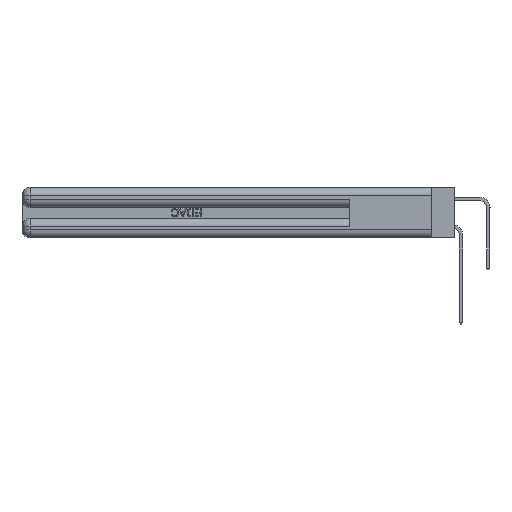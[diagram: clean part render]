
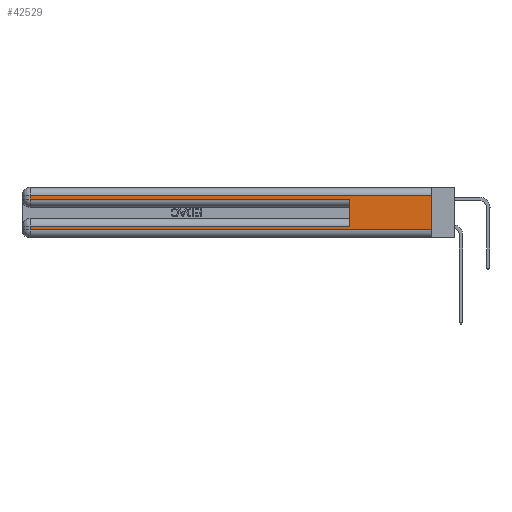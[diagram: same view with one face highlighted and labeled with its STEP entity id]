
A CAD part, left-side view. The second image highlights one B-rep face of the part: STEP entity #42529.
In plain terms, the highlighted planar face has unit normal (-1, 0, 0).
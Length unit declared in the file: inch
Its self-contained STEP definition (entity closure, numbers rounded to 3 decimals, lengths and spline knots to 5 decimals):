
#218 = CARTESIAN_POINT ( 'NONE',  ( 0., 0., 0.06 ) ) ;
#283 = CARTESIAN_POINT ( 'NONE',  ( 0., 0., 0.085 ) ) ;
#600 = CARTESIAN_POINT ( 'NONE',  ( 0., 2.94, 0.285 ) ) ;
#2326 = LINE ( 'NONE', #10565, #32138 ) ;
#2360 = VERTEX_POINT ( 'NONE', #32307 ) ;
#3312 = EDGE_CURVE ( 'NONE', #2360, #39725, #22812, .T. ) ;
#5415 = AXIS2_PLACEMENT_3D ( 'NONE', #45725, #49653, #26412 ) ;
#6500 = CARTESIAN_POINT ( 'NONE',  ( 0., 2.94, 0.31 ) ) ;
#8072 = DIRECTION ( 'NONE',  ( 0., -1., 0. ) ) ;
#8372 = ORIENTED_EDGE ( 'NONE', *, *, #28988, .T. ) ;
#9056 = ORIENTED_EDGE ( 'NONE', *, *, #31127, .T. ) ;
#10244 = CARTESIAN_POINT ( 'NONE',  ( 0., 0.6, 0.285 ) ) ;
#10565 = CARTESIAN_POINT ( 'NONE',  ( 0., 2.94, 0.37 ) ) ;
#11269 = ORIENTED_EDGE ( 'NONE', *, *, #49576, .F. ) ;
#12846 = CARTESIAN_POINT ( 'NONE',  ( 0., 0.6, 0.145 ) ) ;
#13101 = VERTEX_POINT ( 'NONE', #48959 ) ;
#13306 = VECTOR ( 'NONE', #44226, 39.37008 ) ;
#13321 = DIRECTION ( 'NONE',  ( 0., 0., -1. ) ) ;
#14758 = LINE ( 'NONE', #283, #44543 ) ;
#15960 = VECTOR ( 'NONE', #45508, 39.37008 ) ;
#16211 = FACE_OUTER_BOUND ( 'NONE', #19520, .T. ) ;
#17081 = CARTESIAN_POINT ( 'NONE',  ( 0., 2.94, 0.37 ) ) ;
#17182 = LINE ( 'NONE', #33832, #15960 ) ;
#17211 = CARTESIAN_POINT ( 'NONE',  ( 0., 0., 0.37 ) ) ;
#17483 = VECTOR ( 'NONE', #8072, 39.37008 ) ;
#18579 = PLANE ( 'NONE',  #5415 ) ;
#19336 = DIRECTION ( 'NONE',  ( 0., 1., 0. ) ) ;
#19520 = EDGE_LOOP ( 'NONE', ( #33938, #31603, #29012, #8372, #11269, #9056, #35005, #23193 ) ) ;
#20106 = CARTESIAN_POINT ( 'NONE',  ( 0., 2.94, 0.06 ) ) ;
#20500 = EDGE_CURVE ( 'NONE', #38505, #43657, #37856, .T. ) ;
#22812 = LINE ( 'NONE', #30873, #31927 ) ;
#23193 = ORIENTED_EDGE ( 'NONE', *, *, #42039, .T. ) ;
#26412 = DIRECTION ( 'NONE',  ( 0., 0., -1. ) ) ;
#27534 = DIRECTION ( 'NONE',  ( 0., 1., 0. ) ) ;
#28988 = EDGE_CURVE ( 'NONE', #33317, #43287, #17182, .T. ) ;
#29012 = ORIENTED_EDGE ( 'NONE', *, *, #34376, .T. ) ;
#29928 = CARTESIAN_POINT ( 'NONE',  ( 0., 0., 0.06 ) ) ;
#30135 = DIRECTION ( 'NONE',  ( 0., 0., -1. ) ) ;
#30873 = CARTESIAN_POINT ( 'NONE',  ( 0., 0., 0.31 ) ) ;
#31127 = EDGE_CURVE ( 'NONE', #13101, #38505, #14758, .T. ) ;
#31603 = ORIENTED_EDGE ( 'NONE', *, *, #3312, .T. ) ;
#31927 = VECTOR ( 'NONE', #19336, 39.37008 ) ;
#32138 = VECTOR ( 'NONE', #30135, 39.37008 ) ;
#32307 = CARTESIAN_POINT ( 'NONE',  ( 0., 0., 0.31 ) ) ;
#32468 = VECTOR ( 'NONE', #47820, 39.37008 ) ;
#32789 = LINE ( 'NONE', #17211, #13306 ) ;
#33317 = VERTEX_POINT ( 'NONE', #600 ) ;
#33832 = CARTESIAN_POINT ( 'NONE',  ( 0., 0., 0.285 ) ) ;
#33938 = ORIENTED_EDGE ( 'NONE', *, *, #34147, .F. ) ;
#34147 = EDGE_CURVE ( 'NONE', #2360, #45998, #32789, .T. ) ;
#34376 = EDGE_CURVE ( 'NONE', #39725, #33317, #2326, .T. ) ;
#35005 = ORIENTED_EDGE ( 'NONE', *, *, #20500, .T. ) ;
#36633 = VECTOR ( 'NONE', #13321, 39.37008 ) ;
#37856 = LINE ( 'NONE', #17081, #36633 ) ;
#38505 = VERTEX_POINT ( 'NONE', #41247 ) ;
#39725 = VERTEX_POINT ( 'NONE', #6500 ) ;
#41247 = CARTESIAN_POINT ( 'NONE',  ( 0., 2.94, 0.085 ) ) ;
#42039 = EDGE_CURVE ( 'NONE', #43657, #45998, #48475, .T. ) ;
#42529 = ADVANCED_FACE ( 'NONE', ( #16211 ), #18579, .F. ) ;
#42778 = LINE ( 'NONE', #12846, #32468 ) ;
#43287 = VERTEX_POINT ( 'NONE', #10244 ) ;
#43657 = VERTEX_POINT ( 'NONE', #20106 ) ;
#44226 = DIRECTION ( 'NONE',  ( 0., 0., -1. ) ) ;
#44543 = VECTOR ( 'NONE', #27534, 39.37008 ) ;
#45508 = DIRECTION ( 'NONE',  ( 0., -1., 0. ) ) ;
#45725 = CARTESIAN_POINT ( 'NONE',  ( 0., 0., 0.37 ) ) ;
#45998 = VERTEX_POINT ( 'NONE', #29928 ) ;
#47820 = DIRECTION ( 'NONE',  ( 0., 0., 1. ) ) ;
#48475 = LINE ( 'NONE', #218, #17483 ) ;
#48959 = CARTESIAN_POINT ( 'NONE',  ( 0., 0.6, 0.085 ) ) ;
#49576 = EDGE_CURVE ( 'NONE', #13101, #43287, #42778, .T. ) ;
#49653 = DIRECTION ( 'NONE',  ( 1., 0., 0. ) ) ;
